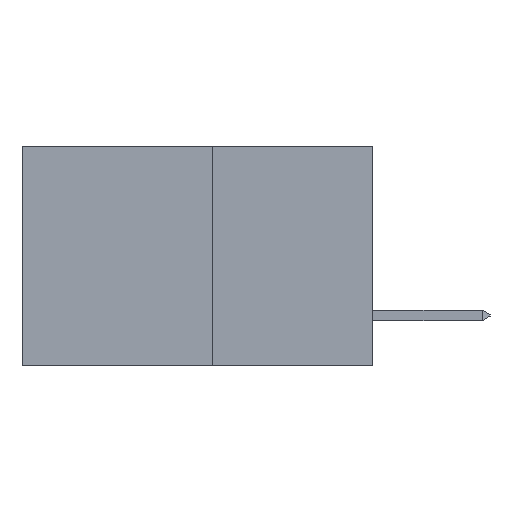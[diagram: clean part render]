
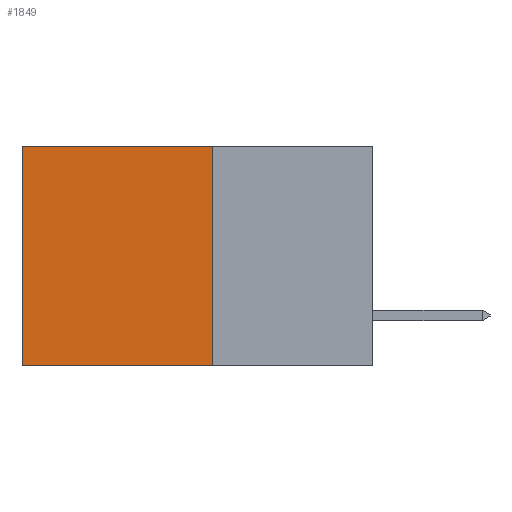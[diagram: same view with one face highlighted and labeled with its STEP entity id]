
A CAD part, left-side view. The second image highlights one B-rep face of the part: STEP entity #1849.
In plain terms, the highlighted planar face has unit normal (-1, 0, 0).
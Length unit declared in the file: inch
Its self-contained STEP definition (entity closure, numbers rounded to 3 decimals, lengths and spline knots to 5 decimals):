
#432 = VERTEX_POINT ( 'NONE', #6597 ) ;
#1151 = DIRECTION ( 'NONE',  ( 0., 1., 0. ) ) ;
#1540 = EDGE_CURVE ( 'NONE', #5870, #432, #10724, .T. ) ;
#1588 = DIRECTION ( 'NONE',  ( 0., 1., 0. ) ) ;
#1600 = CARTESIAN_POINT ( 'NONE',  ( 0.277, 0.27, -0.37 ) ) ;
#1840 = CARTESIAN_POINT ( 'NONE',  ( 0.277, 0.59, -0.37 ) ) ;
#1849 = ADVANCED_FACE ( 'NONE', ( #3606 ), #7844, .F. ) ;
#2081 = CARTESIAN_POINT ( 'NONE',  ( 0.277, 0.59, -0.37 ) ) ;
#2168 = EDGE_CURVE ( 'NONE', #5870, #6494, #4923, .T. ) ;
#2501 = VECTOR ( 'NONE', #4072, 39.37008 ) ;
#2795 = CARTESIAN_POINT ( 'NONE',  ( 0.277, 0.27, 0. ) ) ;
#3018 = EDGE_CURVE ( 'NONE', #6494, #9773, #9708, .T. ) ;
#3310 = ORIENTED_EDGE ( 'NONE', *, *, #3018, .T. ) ;
#3329 = ORIENTED_EDGE ( 'NONE', *, *, #9079, .F. ) ;
#3341 = ORIENTED_EDGE ( 'NONE', *, *, #1540, .F. ) ;
#3356 = ORIENTED_EDGE ( 'NONE', *, *, #2168, .T. ) ;
#3538 = EDGE_LOOP ( 'NONE', ( #3310, #3329, #3341, #3356 ) ) ;
#3606 = FACE_OUTER_BOUND ( 'NONE', #3538, .T. ) ;
#4072 = DIRECTION ( 'NONE',  ( 0., 0., -1. ) ) ;
#4275 = DIRECTION ( 'NONE',  ( 0., 0., -1. ) ) ;
#4657 = VECTOR ( 'NONE', #1151, 39.37008 ) ;
#4923 = LINE ( 'NONE', #9559, #4657 ) ;
#5870 = VERTEX_POINT ( 'NONE', #2795 ) ;
#6296 = LINE ( 'NONE', #1600, #6567 ) ;
#6494 = VERTEX_POINT ( 'NONE', #9852 ) ;
#6567 = VECTOR ( 'NONE', #1588, 39.37008 ) ;
#6597 = CARTESIAN_POINT ( 'NONE',  ( 0.277, 0.27, -0.37 ) ) ;
#7105 = VECTOR ( 'NONE', #9560, 39.37008 ) ;
#7844 = PLANE ( 'NONE',  #8707 ) ;
#8707 = AXIS2_PLACEMENT_3D ( 'NONE', #9782, #10866, #4275 ) ;
#9079 = EDGE_CURVE ( 'NONE', #432, #9773, #6296, .T. ) ;
#9559 = CARTESIAN_POINT ( 'NONE',  ( 0.277, 0.27, 0. ) ) ;
#9560 = DIRECTION ( 'NONE',  ( 0., 0., -1. ) ) ;
#9708 = LINE ( 'NONE', #2081, #7105 ) ;
#9753 = CARTESIAN_POINT ( 'NONE',  ( 0.277, 0.27, -0.37 ) ) ;
#9773 = VERTEX_POINT ( 'NONE', #1840 ) ;
#9782 = CARTESIAN_POINT ( 'NONE',  ( 0.277, 0.27, -0.37 ) ) ;
#9852 = CARTESIAN_POINT ( 'NONE',  ( 0.277, 0.59, 0. ) ) ;
#10724 = LINE ( 'NONE', #9753, #2501 ) ;
#10866 = DIRECTION ( 'NONE',  ( 1., 0., 0. ) ) ;
